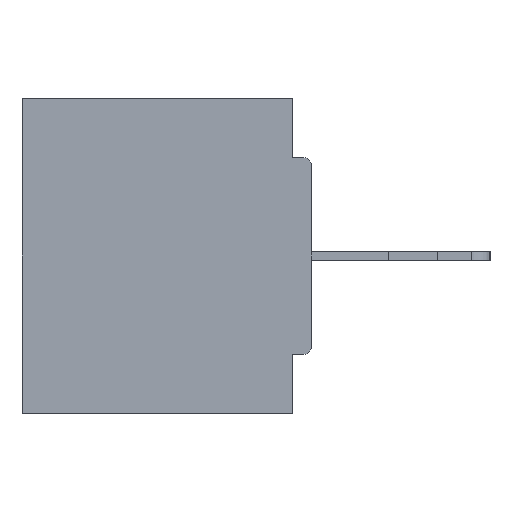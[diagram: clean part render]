
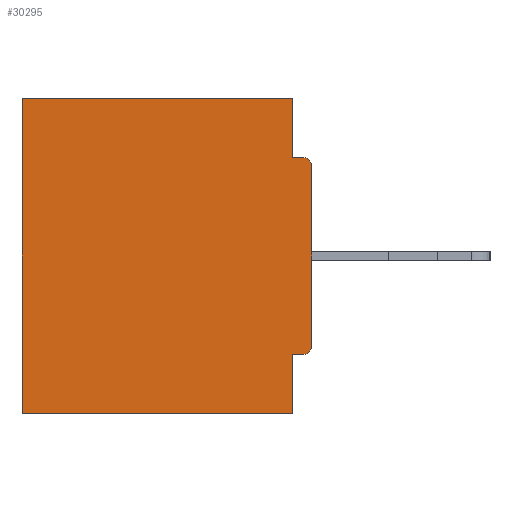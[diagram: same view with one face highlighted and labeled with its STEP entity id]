
A CAD part, left-side view. The second image highlights one B-rep face of the part: STEP entity #30295.
In plain terms, the highlighted planar face has unit normal (-1, 0, 0).
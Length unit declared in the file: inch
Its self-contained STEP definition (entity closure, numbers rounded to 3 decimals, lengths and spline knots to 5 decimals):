
#147 = VERTEX_POINT ( 'NONE', #11205 ) ;
#202 = VERTEX_POINT ( 'NONE', #16925 ) ;
#232 = VERTEX_POINT ( 'NONE', #17819 ) ;
#448 = ORIENTED_EDGE ( 'NONE', *, *, #31033, .F. ) ;
#572 = EDGE_CURVE ( 'NONE', #17031, #232, #12564, .T. ) ;
#833 = CARTESIAN_POINT ( 'NONE',  ( 0.298, 0., -0.0935 ) ) ;
#1626 = CARTESIAN_POINT ( 'NONE',  ( 0.298, 0.031, 0. ) ) ;
#2241 = ORIENTED_EDGE ( 'NONE', *, *, #14754, .T. ) ;
#2290 = VECTOR ( 'NONE', #10846, 39.37008 ) ;
#2509 = ORIENTED_EDGE ( 'NONE', *, *, #15476, .T. ) ;
#2887 = EDGE_CURVE ( 'NONE', #30931, #31344, #26671, .T. ) ;
#2921 = ORIENTED_EDGE ( 'NONE', *, *, #2887, .F. ) ;
#3725 = CARTESIAN_POINT ( 'NONE',  ( 0.298, 0., -0.5 ) ) ;
#4082 = VECTOR ( 'NONE', #19602, 39.37008 ) ;
#4101 = CARTESIAN_POINT ( 'NONE',  ( 0.298, 0., 0. ) ) ;
#4505 = AXIS2_PLACEMENT_3D ( 'NONE', #7185, #24462, #9728 ) ;
#4879 = LINE ( 'NONE', #29089, #4082 ) ;
#5651 = ORIENTED_EDGE ( 'NONE', *, *, #20350, .T. ) ;
#5983 = CARTESIAN_POINT ( 'NONE',  ( 0.298, 0., -0.1085 ) ) ;
#6200 = VECTOR ( 'NONE', #29354, 39.37008 ) ;
#6244 = DIRECTION ( 'NONE',  ( 0., 1., 0. ) ) ;
#6757 = CARTESIAN_POINT ( 'NONE',  ( 0.298, 0., 0. ) ) ;
#7185 = CARTESIAN_POINT ( 'NONE',  ( 0.298, 0.015, -0.1085 ) ) ;
#7804 = ORIENTED_EDGE ( 'NONE', *, *, #30504, .F. ) ;
#8070 = LINE ( 'NONE', #17496, #8848 ) ;
#8848 = VECTOR ( 'NONE', #12509, 39.37008 ) ;
#8939 = LINE ( 'NONE', #13397, #2290 ) ;
#9728 = DIRECTION ( 'NONE',  ( 0., 0., -1. ) ) ;
#9987 = CARTESIAN_POINT ( 'NONE',  ( 0.298, 0.46, 0. ) ) ;
#10800 = ORIENTED_EDGE ( 'NONE', *, *, #15609, .T. ) ;
#10846 = DIRECTION ( 'NONE',  ( 0., 0., -1. ) ) ;
#11000 = CARTESIAN_POINT ( 'NONE',  ( 0.298, 0.46, -0.5 ) ) ;
#11096 = CARTESIAN_POINT ( 'NONE',  ( 0.298, 0.015, -0.3915 ) ) ;
#11163 = AXIS2_PLACEMENT_3D ( 'NONE', #12376, #29411, #14922 ) ;
#11205 = CARTESIAN_POINT ( 'NONE',  ( 0.298, 0.031, -0.5 ) ) ;
#11545 = VERTEX_POINT ( 'NONE', #23792 ) ;
#11673 = ORIENTED_EDGE ( 'NONE', *, *, #16483, .F. ) ;
#11788 = VERTEX_POINT ( 'NONE', #9987 ) ;
#12376 = CARTESIAN_POINT ( 'NONE',  ( 0.298, 0., 0. ) ) ;
#12422 = ORIENTED_EDGE ( 'NONE', *, *, #572, .F. ) ;
#12509 = DIRECTION ( 'NONE',  ( 0., 0., -1. ) ) ;
#12564 = LINE ( 'NONE', #6757, #24808 ) ;
#13397 = CARTESIAN_POINT ( 'NONE',  ( 0.298, 0.46, 0. ) ) ;
#13654 = DIRECTION ( 'NONE',  ( 0., 0., -1. ) ) ;
#14442 = CARTESIAN_POINT ( 'NONE',  ( 0.298, 0.015, -0.0935 ) ) ;
#14754 = EDGE_CURVE ( 'NONE', #11545, #232, #23395, .T. ) ;
#14922 = DIRECTION ( 'NONE',  ( 0., 0., -1. ) ) ;
#15476 = EDGE_CURVE ( 'NONE', #30931, #11788, #30089, .T. ) ;
#15609 = EDGE_CURVE ( 'NONE', #17031, #29093, #31202, .T. ) ;
#15853 = DIRECTION ( 'NONE',  ( 0., -1., 0. ) ) ;
#16483 = EDGE_CURVE ( 'NONE', #147, #24627, #30842, .T. ) ;
#16925 = CARTESIAN_POINT ( 'NONE',  ( 0.298, 0.031, -0.4065 ) ) ;
#17031 = VERTEX_POINT ( 'NONE', #5983 ) ;
#17496 = CARTESIAN_POINT ( 'NONE',  ( 0.298, 0.031, -0.5 ) ) ;
#17819 = CARTESIAN_POINT ( 'NONE',  ( 0.298, 0., -0.3915 ) ) ;
#18107 = EDGE_CURVE ( 'NONE', #31344, #29093, #21707, .T. ) ;
#19602 = DIRECTION ( 'NONE',  ( 0., 1., 0. ) ) ;
#19727 = DIRECTION ( 'NONE',  ( 0., 0., -1. ) ) ;
#19729 = PLANE ( 'NONE',  #11163 ) ;
#20350 = EDGE_CURVE ( 'NONE', #11788, #24627, #8939, .T. ) ;
#21298 = CARTESIAN_POINT ( 'NONE',  ( 0.298, 0.031, -0.0935 ) ) ;
#21707 = LINE ( 'NONE', #833, #28098 ) ;
#22007 = AXIS2_PLACEMENT_3D ( 'NONE', #11096, #28208, #13654 ) ;
#22036 = EDGE_LOOP ( 'NONE', ( #10800, #27883, #2921, #2509, #5651, #11673, #7804, #448, #2241, #12422 ) ) ;
#22435 = FACE_OUTER_BOUND ( 'NONE', #22036, .T. ) ;
#23395 = CIRCLE ( 'NONE', #22007, 0.015 ) ;
#23406 = CARTESIAN_POINT ( 'NONE',  ( 0.298, 0.031, -0.5 ) ) ;
#23792 = CARTESIAN_POINT ( 'NONE',  ( 0.298, 0.015, -0.4065 ) ) ;
#23941 = DIRECTION ( 'NONE',  ( 0., 1., 0. ) ) ;
#24444 = VECTOR ( 'NONE', #6244, 39.37008 ) ;
#24462 = DIRECTION ( 'NONE',  ( -1., 0., 0. ) ) ;
#24627 = VERTEX_POINT ( 'NONE', #11000 ) ;
#24808 = VECTOR ( 'NONE', #19727, 39.37008 ) ;
#26671 = LINE ( 'NONE', #23406, #6200 ) ;
#27854 = VECTOR ( 'NONE', #23941, 39.37008 ) ;
#27883 = ORIENTED_EDGE ( 'NONE', *, *, #18107, .F. ) ;
#28098 = VECTOR ( 'NONE', #15853, 39.37008 ) ;
#28208 = DIRECTION ( 'NONE',  ( -1., 0., 0. ) ) ;
#29089 = CARTESIAN_POINT ( 'NONE',  ( 0.298, 0., -0.4065 ) ) ;
#29093 = VERTEX_POINT ( 'NONE', #14442 ) ;
#29354 = DIRECTION ( 'NONE',  ( 0., 0., -1. ) ) ;
#29411 = DIRECTION ( 'NONE',  ( 1., 0., 0. ) ) ;
#30089 = LINE ( 'NONE', #4101, #27854 ) ;
#30295 = ADVANCED_FACE ( 'NONE', ( #22435 ), #19729, .F. ) ;
#30504 = EDGE_CURVE ( 'NONE', #202, #147, #8070, .T. ) ;
#30842 = LINE ( 'NONE', #3725, #24444 ) ;
#30931 = VERTEX_POINT ( 'NONE', #1626 ) ;
#31033 = EDGE_CURVE ( 'NONE', #11545, #202, #4879, .T. ) ;
#31202 = CIRCLE ( 'NONE', #4505, 0.015 ) ;
#31344 = VERTEX_POINT ( 'NONE', #21298 ) ;
